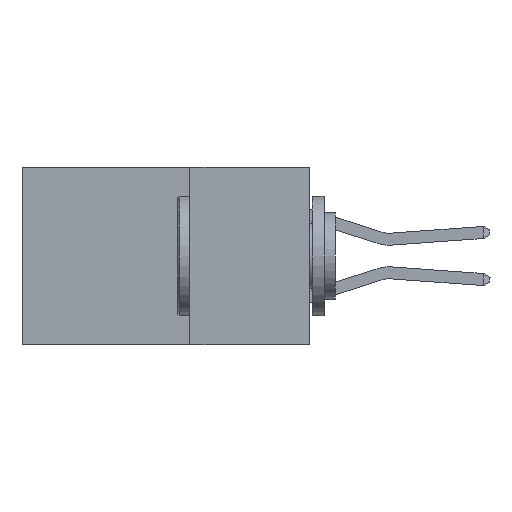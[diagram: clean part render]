
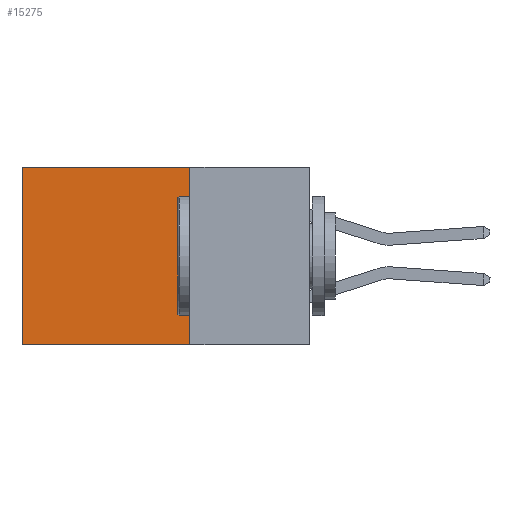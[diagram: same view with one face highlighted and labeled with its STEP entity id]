
A CAD part, left-side view. The second image highlights one B-rep face of the part: STEP entity #15275.
In plain terms, the highlighted planar face has unit normal (-1, 0, 0).
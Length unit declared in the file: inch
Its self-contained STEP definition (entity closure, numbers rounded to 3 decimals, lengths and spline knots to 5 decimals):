
#723 = DIRECTION ( 'NONE',  ( 1., 0., 0. ) ) ;
#901 = LINE ( 'NONE', #21182, #6110 ) ;
#916 = PLANE ( 'NONE',  #7380 ) ;
#3359 = VERTEX_POINT ( 'NONE', #14661 ) ;
#3822 = CARTESIAN_POINT ( 'NONE',  ( 0.298, 0.25, -0.37 ) ) ;
#4686 = EDGE_CURVE ( 'NONE', #23705, #12444, #19781, .T. ) ;
#5163 = CARTESIAN_POINT ( 'NONE',  ( 0.298, 0.25, -0.37 ) ) ;
#5481 = CARTESIAN_POINT ( 'NONE',  ( 0.298, 0.25, 0. ) ) ;
#5697 = LINE ( 'NONE', #17014, #14399 ) ;
#6110 = VECTOR ( 'NONE', #19032, 39.37008 ) ;
#6534 = CARTESIAN_POINT ( 'NONE',  ( 0.298, 0.25, 0. ) ) ;
#6764 = EDGE_CURVE ( 'NONE', #3359, #15540, #901, .T. ) ;
#7380 = AXIS2_PLACEMENT_3D ( 'NONE', #5481, #723, #14326 ) ;
#8312 = VECTOR ( 'NONE', #10643, 39.37008 ) ;
#10643 = DIRECTION ( 'NONE',  ( 0., 0., -1. ) ) ;
#12163 = ORIENTED_EDGE ( 'NONE', *, *, #14729, .T. ) ;
#12444 = VERTEX_POINT ( 'NONE', #5163 ) ;
#12663 = FACE_OUTER_BOUND ( 'NONE', #15391, .T. ) ;
#12865 = DIRECTION ( 'NONE',  ( 0., 1., 0. ) ) ;
#14326 = DIRECTION ( 'NONE',  ( 0., 0., -1. ) ) ;
#14331 = ORIENTED_EDGE ( 'NONE', *, *, #6764, .T. ) ;
#14399 = VECTOR ( 'NONE', #12865, 39.37008 ) ;
#14661 = CARTESIAN_POINT ( 'NONE',  ( 0.298, 0.6, 0. ) ) ;
#14699 = DIRECTION ( 'NONE',  ( 0., 1., 0. ) ) ;
#14729 = EDGE_CURVE ( 'NONE', #23705, #3359, #5697, .T. ) ;
#15275 = ADVANCED_FACE ( 'NONE', ( #12663 ), #916, .F. ) ;
#15391 = EDGE_LOOP ( 'NONE', ( #14331, #15744, #17201, #12163 ) ) ;
#15540 = VERTEX_POINT ( 'NONE', #23900 ) ;
#15744 = ORIENTED_EDGE ( 'NONE', *, *, #17636, .F. ) ;
#17014 = CARTESIAN_POINT ( 'NONE',  ( 0.298, 0.25, 0. ) ) ;
#17201 = ORIENTED_EDGE ( 'NONE', *, *, #4686, .F. ) ;
#17636 = EDGE_CURVE ( 'NONE', #12444, #15540, #25040, .T. ) ;
#19032 = DIRECTION ( 'NONE',  ( 0., 0., -1. ) ) ;
#19480 = VECTOR ( 'NONE', #14699, 39.37008 ) ;
#19781 = LINE ( 'NONE', #23394, #8312 ) ;
#21182 = CARTESIAN_POINT ( 'NONE',  ( 0.298, 0.6, 0. ) ) ;
#23394 = CARTESIAN_POINT ( 'NONE',  ( 0.298, 0.25, 0. ) ) ;
#23705 = VERTEX_POINT ( 'NONE', #6534 ) ;
#23900 = CARTESIAN_POINT ( 'NONE',  ( 0.298, 0.6, -0.37 ) ) ;
#25040 = LINE ( 'NONE', #3822, #19480 ) ;
